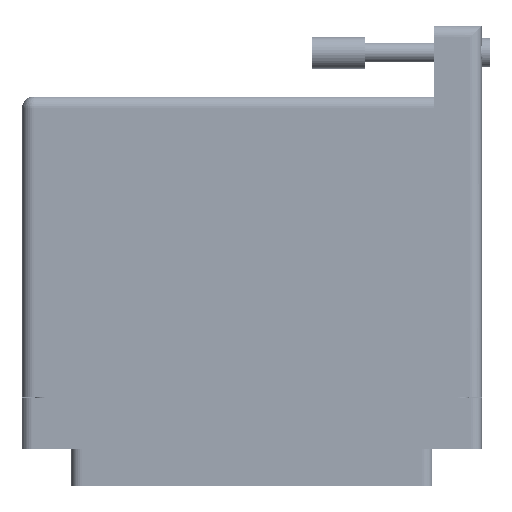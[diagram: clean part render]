
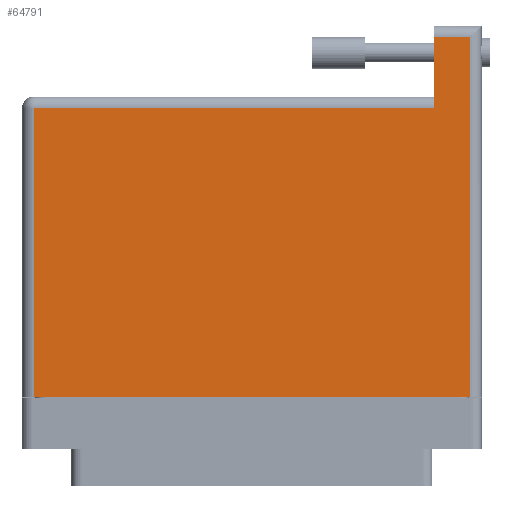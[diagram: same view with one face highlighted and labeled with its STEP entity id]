
A CAD part, front view. The second image highlights one B-rep face of the part: STEP entity #64791.
In plain terms, the highlighted face is planar.
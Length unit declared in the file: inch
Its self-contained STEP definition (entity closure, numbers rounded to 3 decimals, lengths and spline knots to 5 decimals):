
#1036 = ORIENTED_EDGE ( 'NONE', *, *, #54704, .T. ) ;
#3611 = DIRECTION ( 'NONE',  ( 0., 0., -1. ) ) ;
#6445 = EDGE_CURVE ( 'NONE', #26126, #69346, #22285, .T. ) ;
#6486 = VECTOR ( 'NONE', #38462, 39.37008 ) ;
#6541 = CARTESIAN_POINT ( 'NONE',  ( 1.079, 2.095, 0.617 ) ) ;
#8710 = VECTOR ( 'NONE', #42654, 39.37008 ) ;
#8828 = CARTESIAN_POINT ( 'NONE',  ( -1.359, 1.675, 0.617 ) ) ;
#10124 = EDGE_LOOP ( 'NONE', ( #61871, #13112, #55429, #14603, #1036, #43249 ) ) ;
#11337 = CARTESIAN_POINT ( 'NONE',  ( 1.289, 2.025, 0.617 ) ) ;
#12987 = EDGE_CURVE ( 'NONE', #39369, #35167, #29487, .T. ) ;
#13112 = ORIENTED_EDGE ( 'NONE', *, *, #27760, .T. ) ;
#14056 = LINE ( 'NONE', #65905, #41123 ) ;
#14603 = ORIENTED_EDGE ( 'NONE', *, *, #52850, .T. ) ;
#18299 = VECTOR ( 'NONE', #62112, 39.37008 ) ;
#19181 = PLANE ( 'NONE',  #22222 ) ;
#21170 = CARTESIAN_POINT ( 'NONE',  ( -1.289, 1.605, 0.617 ) ) ;
#22222 = AXIS2_PLACEMENT_3D ( 'NONE', #8828, #3611, #25026 ) ;
#22285 = LINE ( 'NONE', #41970, #8710 ) ;
#25026 = DIRECTION ( 'NONE',  ( -1., 0., 0. ) ) ;
#26126 = VERTEX_POINT ( 'NONE', #37195 ) ;
#27255 = LINE ( 'NONE', #54267, #47609 ) ;
#27760 = EDGE_CURVE ( 'NONE', #49728, #26126, #14056, .T. ) ;
#29487 = LINE ( 'NONE', #6541, #6486 ) ;
#32285 = EDGE_CURVE ( 'NONE', #35167, #49728, #61937, .T. ) ;
#32622 = LINE ( 'NONE', #36059, #18299 ) ;
#32671 = DIRECTION ( 'NONE',  ( -1., 0., 0. ) ) ;
#34092 = FACE_OUTER_BOUND ( 'NONE', #10124, .T. ) ;
#34522 = VERTEX_POINT ( 'NONE', #11337 ) ;
#35167 = VERTEX_POINT ( 'NONE', #63157 ) ;
#36059 = CARTESIAN_POINT ( 'NONE',  ( 1.289, 2.095, 0.617 ) ) ;
#36183 = CARTESIAN_POINT ( 'NONE',  ( 1.079, 2.025, 0.617 ) ) ;
#37195 = CARTESIAN_POINT ( 'NONE',  ( -1.289, -0.1, 0.617 ) ) ;
#38462 = DIRECTION ( 'NONE',  ( 0., -1., 0. ) ) ;
#38912 = DIRECTION ( 'NONE',  ( 0., -1., 0. ) ) ;
#39369 = VERTEX_POINT ( 'NONE', #36183 ) ;
#41123 = VECTOR ( 'NONE', #38912, 39.37008 ) ;
#41970 = CARTESIAN_POINT ( 'NONE',  ( -1.359, -0.1, 0.617 ) ) ;
#42466 = CARTESIAN_POINT ( 'NONE',  ( -1.359, 1.605, 0.617 ) ) ;
#42654 = DIRECTION ( 'NONE',  ( 1., 0., 0. ) ) ;
#43249 = ORIENTED_EDGE ( 'NONE', *, *, #12987, .T. ) ;
#47609 = VECTOR ( 'NONE', #32671, 39.37008 ) ;
#49728 = VERTEX_POINT ( 'NONE', #21170 ) ;
#52850 = EDGE_CURVE ( 'NONE', #69346, #34522, #32622, .T. ) ;
#54267 = CARTESIAN_POINT ( 'NONE',  ( -1.359, 2.025, 0.617 ) ) ;
#54704 = EDGE_CURVE ( 'NONE', #34522, #39369, #27255, .T. ) ;
#55429 = ORIENTED_EDGE ( 'NONE', *, *, #6445, .T. ) ;
#61871 = ORIENTED_EDGE ( 'NONE', *, *, #32285, .T. ) ;
#61937 = LINE ( 'NONE', #42466, #66212 ) ;
#62112 = DIRECTION ( 'NONE',  ( 0., 1., 0. ) ) ;
#63157 = CARTESIAN_POINT ( 'NONE',  ( 1.079, 1.605, 0.617 ) ) ;
#64791 = ADVANCED_FACE ( 'NONE', ( #34092 ), #19181, .F. ) ;
#65905 = CARTESIAN_POINT ( 'NONE',  ( -1.289, -0.1, 0.617 ) ) ;
#66212 = VECTOR ( 'NONE', #69273, 39.37008 ) ;
#67409 = CARTESIAN_POINT ( 'NONE',  ( 1.289, -0.1, 0.617 ) ) ;
#69273 = DIRECTION ( 'NONE',  ( -1., 0., 0. ) ) ;
#69346 = VERTEX_POINT ( 'NONE', #67409 ) ;
